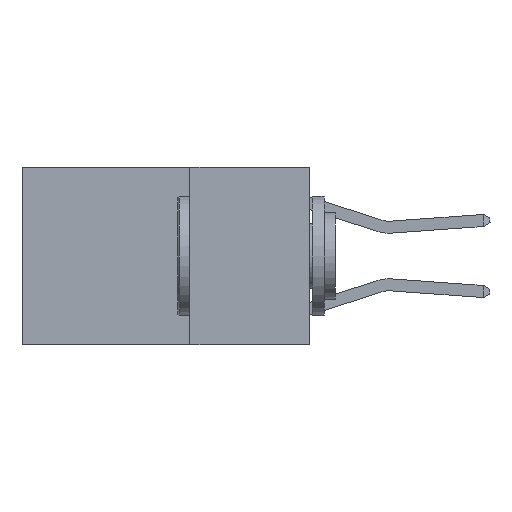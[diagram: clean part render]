
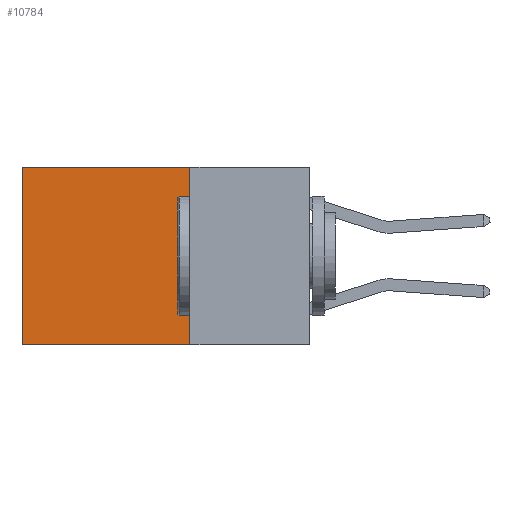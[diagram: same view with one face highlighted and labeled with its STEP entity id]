
A CAD part, left-side view. The second image highlights one B-rep face of the part: STEP entity #10784.
In plain terms, the highlighted planar face has unit normal (-1, 0, 0).
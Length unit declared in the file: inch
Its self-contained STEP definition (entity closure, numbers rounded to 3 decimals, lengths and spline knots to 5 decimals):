
#262 = EDGE_CURVE ( 'NONE', #12802, #15913, #15794, .T. ) ;
#462 = CARTESIAN_POINT ( 'NONE',  ( 0.2625, 0.25, 0. ) ) ;
#683 = CARTESIAN_POINT ( 'NONE',  ( 0.2625, 0.25, -0.37 ) ) ;
#851 = CARTESIAN_POINT ( 'NONE',  ( 0.2625, 0.6, 0. ) ) ;
#1403 = LINE ( 'NONE', #851, #14054 ) ;
#1530 = CARTESIAN_POINT ( 'NONE',  ( 0.2625, 0.25, 0. ) ) ;
#2161 = DIRECTION ( 'NONE',  ( 0., 0., -1. ) ) ;
#2794 = CARTESIAN_POINT ( 'NONE',  ( 0.2625, 0.25, 0. ) ) ;
#3373 = EDGE_CURVE ( 'NONE', #10705, #15913, #1403, .T. ) ;
#3551 = ORIENTED_EDGE ( 'NONE', *, *, #4835, .F. ) ;
#3885 = CARTESIAN_POINT ( 'NONE',  ( 0.2625, 0.25, 0. ) ) ;
#4088 = DIRECTION ( 'NONE',  ( 0., 1., 0. ) ) ;
#4835 = EDGE_CURVE ( 'NONE', #6469, #12802, #15896, .T. ) ;
#5253 = DIRECTION ( 'NONE',  ( 0., 0., -1. ) ) ;
#6154 = VECTOR ( 'NONE', #4088, 39.37008 ) ;
#6469 = VERTEX_POINT ( 'NONE', #2794 ) ;
#6699 = ORIENTED_EDGE ( 'NONE', *, *, #3373, .T. ) ;
#7138 = ORIENTED_EDGE ( 'NONE', *, *, #15123, .T. ) ;
#7763 = CARTESIAN_POINT ( 'NONE',  ( 0.2625, 0.25, -0.37 ) ) ;
#8438 = DIRECTION ( 'NONE',  ( 0., 0., -1. ) ) ;
#8521 = VECTOR ( 'NONE', #9441, 39.37008 ) ;
#9441 = DIRECTION ( 'NONE',  ( 0., 1., 0. ) ) ;
#10066 = ORIENTED_EDGE ( 'NONE', *, *, #262, .F. ) ;
#10318 = VECTOR ( 'NONE', #8438, 39.37008 ) ;
#10705 = VERTEX_POINT ( 'NONE', #16065 ) ;
#10784 = ADVANCED_FACE ( 'NONE', ( #14127 ), #14981, .F. ) ;
#11313 = LINE ( 'NONE', #1530, #8521 ) ;
#11379 = AXIS2_PLACEMENT_3D ( 'NONE', #3885, #12684, #5253 ) ;
#12684 = DIRECTION ( 'NONE',  ( 1., 0., 0. ) ) ;
#12802 = VERTEX_POINT ( 'NONE', #683 ) ;
#12882 = CARTESIAN_POINT ( 'NONE',  ( 0.2625, 0.6, -0.37 ) ) ;
#13686 = EDGE_LOOP ( 'NONE', ( #6699, #10066, #3551, #7138 ) ) ;
#14054 = VECTOR ( 'NONE', #2161, 39.37008 ) ;
#14127 = FACE_OUTER_BOUND ( 'NONE', #13686, .T. ) ;
#14981 = PLANE ( 'NONE',  #11379 ) ;
#15123 = EDGE_CURVE ( 'NONE', #6469, #10705, #11313, .T. ) ;
#15794 = LINE ( 'NONE', #7763, #6154 ) ;
#15896 = LINE ( 'NONE', #462, #10318 ) ;
#15913 = VERTEX_POINT ( 'NONE', #12882 ) ;
#16065 = CARTESIAN_POINT ( 'NONE',  ( 0.2625, 0.6, 0. ) ) ;
